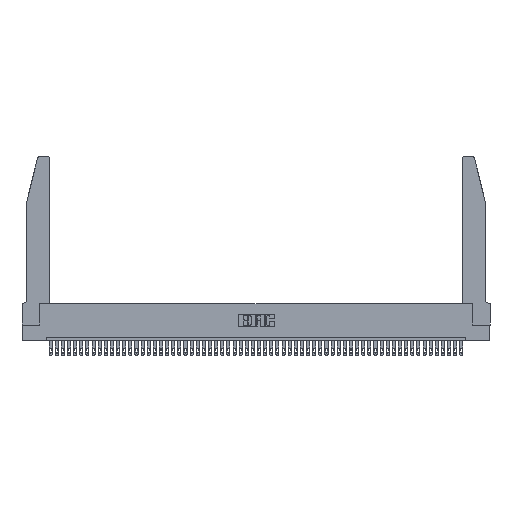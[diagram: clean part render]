
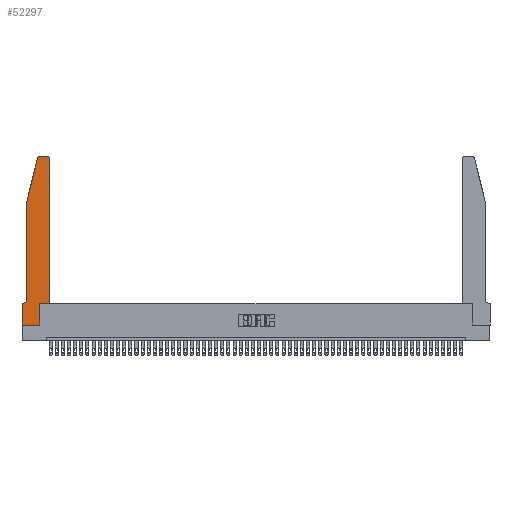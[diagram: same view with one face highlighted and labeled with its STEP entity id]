
A CAD part, top view. The second image highlights one B-rep face of the part: STEP entity #52297.
In plain terms, the highlighted planar face has unit normal (0, 0, 1).
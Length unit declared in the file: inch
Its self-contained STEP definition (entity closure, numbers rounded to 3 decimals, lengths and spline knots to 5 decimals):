
#1409 = DIRECTION ( 'NONE',  ( 0., 0., -1. ) ) ;
#1701 = EDGE_CURVE ( 'NONE', #29514, #42522, #32311, .T. ) ;
#1934 = CARTESIAN_POINT ( 'NONE',  ( 0., 0., 0.37 ) ) ;
#2271 = EDGE_CURVE ( 'NONE', #23830, #29514, #11315, .T. ) ;
#2367 = VERTEX_POINT ( 'NONE', #32939 ) ;
#2663 = EDGE_CURVE ( 'NONE', #42522, #2367, #50556, .T. ) ;
#2724 = LINE ( 'NONE', #51628, #15952 ) ;
#3064 = ORIENTED_EDGE ( 'NONE', *, *, #48895, .T. ) ;
#3779 = CARTESIAN_POINT ( 'NONE',  ( 0.2605, 2.75, 0.37 ) ) ;
#4079 = CARTESIAN_POINT ( 'NONE',  ( 0.4505, 0.35, 0.37 ) ) ;
#4514 = ORIENTED_EDGE ( 'NONE', *, *, #17712, .T. ) ;
#4969 = ORIENTED_EDGE ( 'NONE', *, *, #26431, .T. ) ;
#5219 = ORIENTED_EDGE ( 'NONE', *, *, #2663, .T. ) ;
#5895 = DIRECTION ( 'NONE',  ( -0.239, -0.971, 0. ) ) ;
#6564 = VERTEX_POINT ( 'NONE', #40108 ) ;
#7468 = EDGE_LOOP ( 'NONE', ( #8095, #14667, #5219, #13285, #40168, #13293, #39303, #4969, #19639, #3064, #47855, #4514 ) ) ;
#8095 = ORIENTED_EDGE ( 'NONE', *, *, #2271, .T. ) ;
#8148 = AXIS2_PLACEMENT_3D ( 'NONE', #11819, #12149, #28465 ) ;
#9893 = CARTESIAN_POINT ( 'NONE',  ( 0.4505, 0.35, 0.37 ) ) ;
#10392 = CARTESIAN_POINT ( 'NONE',  ( 0.0755, 0.42, 0.37 ) ) ;
#10551 = CARTESIAN_POINT ( 'NONE',  ( 0., 0., 0.37 ) ) ;
#11315 = LINE ( 'NONE', #3779, #42296 ) ;
#11819 = CARTESIAN_POINT ( 'NONE',  ( 0., 0.35, 0.37 ) ) ;
#12149 = DIRECTION ( 'NONE',  ( 0., 0., 1. ) ) ;
#12997 = CARTESIAN_POINT ( 'NONE',  ( 0.284, 2.75, 0.37 ) ) ;
#13044 = VERTEX_POINT ( 'NONE', #37143 ) ;
#13285 = ORIENTED_EDGE ( 'NONE', *, *, #44915, .T. ) ;
#13293 = ORIENTED_EDGE ( 'NONE', *, *, #46183, .T. ) ;
#13637 = EDGE_CURVE ( 'NONE', #25568, #6564, #31014, .T. ) ;
#14344 = DIRECTION ( 'NONE',  ( 1., 0., 0. ) ) ;
#14667 = ORIENTED_EDGE ( 'NONE', *, *, #1701, .T. ) ;
#14711 = CARTESIAN_POINT ( 'NONE',  ( 0.4505, 0.35, 0.37 ) ) ;
#15853 = PLANE ( 'NONE',  #8148 ) ;
#15952 = VECTOR ( 'NONE', #44011, 39.37008 ) ;
#17264 = DIRECTION ( 'NONE',  ( -1., 0., 0. ) ) ;
#17566 = LINE ( 'NONE', #26568, #18249 ) ;
#17712 = EDGE_CURVE ( 'NONE', #6564, #23830, #27398, .T. ) ;
#18249 = VECTOR ( 'NONE', #38396, 39.37008 ) ;
#18797 = EDGE_CURVE ( 'NONE', #20864, #40181, #46248, .T. ) ;
#19542 = CARTESIAN_POINT ( 'NONE',  ( 0., 0.35, 0.37 ) ) ;
#19639 = ORIENTED_EDGE ( 'NONE', *, *, #39271, .T. ) ;
#20271 = EDGE_CURVE ( 'NONE', #22624, #44719, #27128, .T. ) ;
#20274 = FACE_OUTER_BOUND ( 'NONE', #7468, .T. ) ;
#20738 = AXIS2_PLACEMENT_3D ( 'NONE', #32271, #32739, #36638 ) ;
#20864 = VERTEX_POINT ( 'NONE', #19542 ) ;
#22373 = DIRECTION ( 'NONE',  ( 0., -1., 0. ) ) ;
#22577 = LINE ( 'NONE', #14711, #23229 ) ;
#22618 = CARTESIAN_POINT ( 'NONE',  ( 0.25487, 2.72718, 0.37 ) ) ;
#22624 = VERTEX_POINT ( 'NONE', #10392 ) ;
#23229 = VECTOR ( 'NONE', #14344, 39.37008 ) ;
#23830 = VERTEX_POINT ( 'NONE', #27845 ) ;
#23950 = AXIS2_PLACEMENT_3D ( 'NONE', #37668, #1409, #17264 ) ;
#24181 = AXIS2_PLACEMENT_3D ( 'NONE', #37854, #29373, #49709 ) ;
#25555 = LINE ( 'NONE', #28820, #51595 ) ;
#25568 = VERTEX_POINT ( 'NONE', #9893 ) ;
#25990 = VECTOR ( 'NONE', #22373, 39.37008 ) ;
#26431 = EDGE_CURVE ( 'NONE', #40181, #13044, #43616, .T. ) ;
#26568 = CARTESIAN_POINT ( 'NONE',  ( 0.2865, 0.35, 0.37 ) ) ;
#27128 = CIRCLE ( 'NONE', #23950, 0.07 ) ;
#27178 = CARTESIAN_POINT ( 'NONE',  ( 0., 0., 0.37 ) ) ;
#27398 = CIRCLE ( 'NONE', #24181, 0.03 ) ;
#27845 = CARTESIAN_POINT ( 'NONE',  ( 0.4205, 2.75, 0.37 ) ) ;
#28465 = DIRECTION ( 'NONE',  ( 1., 0., 0. ) ) ;
#28820 = CARTESIAN_POINT ( 'NONE',  ( 0.0755, 2., 0.37 ) ) ;
#29373 = DIRECTION ( 'NONE',  ( 0., 0., 1. ) ) ;
#29514 = VERTEX_POINT ( 'NONE', #12997 ) ;
#30896 = CARTESIAN_POINT ( 'NONE',  ( 0.2865, 0.35, 0.37 ) ) ;
#31014 = LINE ( 'NONE', #4079, #37908 ) ;
#31281 = VERTEX_POINT ( 'NONE', #30896 ) ;
#31907 = CARTESIAN_POINT ( 'NONE',  ( 0.0055, 0.35, 0.37 ) ) ;
#32271 = CARTESIAN_POINT ( 'NONE',  ( 0.284, 2.72, 0.37 ) ) ;
#32311 = CIRCLE ( 'NONE', #20738, 0.03 ) ;
#32739 = DIRECTION ( 'NONE',  ( 0., 0., 1. ) ) ;
#32939 = CARTESIAN_POINT ( 'NONE',  ( 0.0755, 2., 0.37 ) ) ;
#36638 = DIRECTION ( 'NONE',  ( 1., 0., 0. ) ) ;
#37143 = CARTESIAN_POINT ( 'NONE',  ( 0.2865, 0., 0.37 ) ) ;
#37668 = CARTESIAN_POINT ( 'NONE',  ( 0.0055, 0.42, 0.37 ) ) ;
#37854 = CARTESIAN_POINT ( 'NONE',  ( 0.4205, 2.72, 0.37 ) ) ;
#37908 = VECTOR ( 'NONE', #47219, 39.37008 ) ;
#38396 = DIRECTION ( 'NONE',  ( 0., 1., 0. ) ) ;
#38510 = VECTOR ( 'NONE', #5895, 39.37008 ) ;
#39271 = EDGE_CURVE ( 'NONE', #13044, #31281, #17566, .T. ) ;
#39303 = ORIENTED_EDGE ( 'NONE', *, *, #18797, .T. ) ;
#40108 = CARTESIAN_POINT ( 'NONE',  ( 0.4505, 2.72, 0.37 ) ) ;
#40168 = ORIENTED_EDGE ( 'NONE', *, *, #20271, .T. ) ;
#40181 = VERTEX_POINT ( 'NONE', #27178 ) ;
#40862 = DIRECTION ( 'NONE',  ( 0., -1., 0. ) ) ;
#41928 = DIRECTION ( 'NONE',  ( 1., 0., 0. ) ) ;
#42296 = VECTOR ( 'NONE', #49137, 39.37008 ) ;
#42522 = VERTEX_POINT ( 'NONE', #22618 ) ;
#43616 = LINE ( 'NONE', #10551, #44841 ) ;
#44011 = DIRECTION ( 'NONE',  ( -1., 0., 0. ) ) ;
#44719 = VERTEX_POINT ( 'NONE', #31907 ) ;
#44841 = VECTOR ( 'NONE', #41928, 39.37008 ) ;
#44915 = EDGE_CURVE ( 'NONE', #2367, #22624, #25555, .T. ) ;
#46183 = EDGE_CURVE ( 'NONE', #44719, #20864, #2724, .T. ) ;
#46232 = CARTESIAN_POINT ( 'NONE',  ( 0.0755, 2., 0.37 ) ) ;
#46248 = LINE ( 'NONE', #1934, #25990 ) ;
#47219 = DIRECTION ( 'NONE',  ( 0., 1., 0. ) ) ;
#47855 = ORIENTED_EDGE ( 'NONE', *, *, #13637, .T. ) ;
#48895 = EDGE_CURVE ( 'NONE', #31281, #25568, #22577, .T. ) ;
#49137 = DIRECTION ( 'NONE',  ( -1., 0., 0. ) ) ;
#49709 = DIRECTION ( 'NONE',  ( 1., 0., 0. ) ) ;
#50556 = LINE ( 'NONE', #46232, #38510 ) ;
#51595 = VECTOR ( 'NONE', #40862, 39.37008 ) ;
#51628 = CARTESIAN_POINT ( 'NONE',  ( 0.0755, 0.35, 0.37 ) ) ;
#52297 = ADVANCED_FACE ( 'NONE', ( #20274 ), #15853, .T. ) ;
